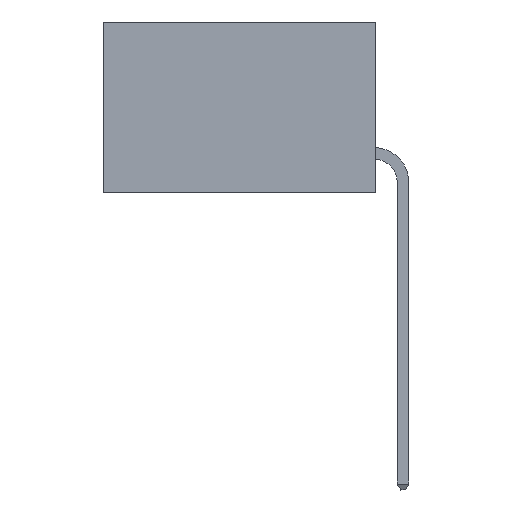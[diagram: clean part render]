
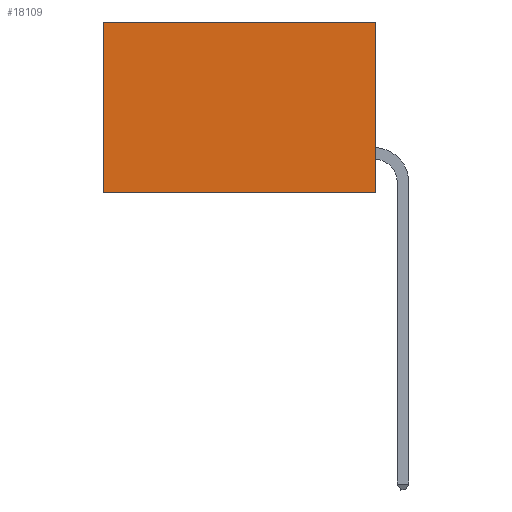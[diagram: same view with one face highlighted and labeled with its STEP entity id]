
A CAD part, left-side view. The second image highlights one B-rep face of the part: STEP entity #18109.
In plain terms, the highlighted planar face has unit normal (-1, 0, 0).
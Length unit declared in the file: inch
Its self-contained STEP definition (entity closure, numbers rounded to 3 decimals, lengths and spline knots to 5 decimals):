
#140 = LINE ( 'NONE', #7484, #13029 ) ;
#233 = VERTEX_POINT ( 'NONE', #14335 ) ;
#1330 = VERTEX_POINT ( 'NONE', #20216 ) ;
#1595 = VERTEX_POINT ( 'NONE', #11369 ) ;
#1670 = ORIENTED_EDGE ( 'NONE', *, *, #3380, .T. ) ;
#2934 = DIRECTION ( 'NONE',  ( 0., 0., -1. ) ) ;
#3150 = CARTESIAN_POINT ( 'NONE',  ( 0.277, 0., 0. ) ) ;
#3380 = EDGE_CURVE ( 'NONE', #15374, #233, #16438, .T. ) ;
#3745 = ORIENTED_EDGE ( 'NONE', *, *, #7291, .T. ) ;
#4005 = ORIENTED_EDGE ( 'NONE', *, *, #14705, .F. ) ;
#4237 = LINE ( 'NONE', #8421, #16428 ) ;
#4593 = LINE ( 'NONE', #14159, #13098 ) ;
#6533 = EDGE_LOOP ( 'NONE', ( #3745, #7322, #4005, #1670 ) ) ;
#7291 = EDGE_CURVE ( 'NONE', #233, #1595, #140, .T. ) ;
#7322 = ORIENTED_EDGE ( 'NONE', *, *, #18845, .F. ) ;
#7484 = CARTESIAN_POINT ( 'NONE',  ( 0.277, 0.59, -0.37 ) ) ;
#7534 = DIRECTION ( 'NONE',  ( 0., 0., -1. ) ) ;
#7984 = CARTESIAN_POINT ( 'NONE',  ( 0.277, 0., 0. ) ) ;
#8238 = DIRECTION ( 'NONE',  ( 1., 0., 0. ) ) ;
#8421 = CARTESIAN_POINT ( 'NONE',  ( 0.277, 0., -0.37 ) ) ;
#8899 = AXIS2_PLACEMENT_3D ( 'NONE', #14498, #8238, #19141 ) ;
#11369 = CARTESIAN_POINT ( 'NONE',  ( 0.277, 0.59, -0.37 ) ) ;
#12275 = VECTOR ( 'NONE', #14002, 39.37008 ) ;
#13029 = VECTOR ( 'NONE', #7534, 39.37008 ) ;
#13098 = VECTOR ( 'NONE', #2934, 39.37008 ) ;
#14002 = DIRECTION ( 'NONE',  ( 0., 1., 0. ) ) ;
#14159 = CARTESIAN_POINT ( 'NONE',  ( 0.277, 0., -0.37 ) ) ;
#14335 = CARTESIAN_POINT ( 'NONE',  ( 0.277, 0.59, 0. ) ) ;
#14498 = CARTESIAN_POINT ( 'NONE',  ( 0.277, 0., -0.37 ) ) ;
#14705 = EDGE_CURVE ( 'NONE', #15374, #1330, #4593, .T. ) ;
#15374 = VERTEX_POINT ( 'NONE', #7984 ) ;
#16428 = VECTOR ( 'NONE', #19318, 39.37008 ) ;
#16438 = LINE ( 'NONE', #3150, #12275 ) ;
#17541 = PLANE ( 'NONE',  #8899 ) ;
#18109 = ADVANCED_FACE ( 'NONE', ( #20437 ), #17541, .F. ) ;
#18845 = EDGE_CURVE ( 'NONE', #1330, #1595, #4237, .T. ) ;
#19141 = DIRECTION ( 'NONE',  ( 0., 0., -1. ) ) ;
#19318 = DIRECTION ( 'NONE',  ( 0., 1., 0. ) ) ;
#20216 = CARTESIAN_POINT ( 'NONE',  ( 0.277, 0., -0.37 ) ) ;
#20437 = FACE_OUTER_BOUND ( 'NONE', #6533, .T. ) ;
